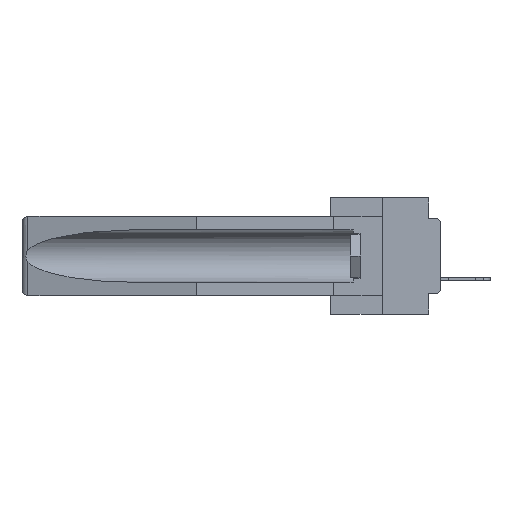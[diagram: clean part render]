
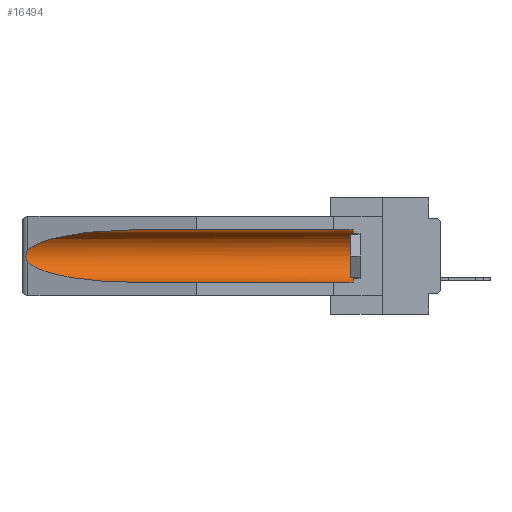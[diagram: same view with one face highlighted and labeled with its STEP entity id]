
A CAD part, left-side view. The second image highlights one B-rep face of the part: STEP entity #16494.
In plain terms, the highlighted cylindrical face has radius 2.857 mm (diameter 5.715 mm), a partial arc.
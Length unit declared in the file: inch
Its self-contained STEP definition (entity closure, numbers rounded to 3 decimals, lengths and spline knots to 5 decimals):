
#127 = CARTESIAN_POINT ( 'NONE',  ( 0.155, 1.07973, -0.284 ) ) ;
#225 = CARTESIAN_POINT ( 'NONE',  ( 0.2673, 1.53269, -0.17917 ) ) ;
#530 = CARTESIAN_POINT ( 'NONE',  ( 0.155, -0.30754, -0.284 ) ) ;
#1042 = ORIENTED_EDGE ( 'NONE', *, *, #26221, .T. ) ;
#1314 = CARTESIAN_POINT ( 'NONE',  ( 0.155, 1.07973, -0.059 ) ) ;
#2080 = ORIENTED_EDGE ( 'NONE', *, *, #26240, .T. ) ;
#2607 = DIRECTION ( 'NONE',  ( 0., 1., 0. ) ) ;
#2804 = CARTESIAN_POINT ( 'NONE',  ( 0.26655, 1.53094, -0.18657 ) ) ;
#3484 = AXIS2_PLACEMENT_3D ( 'NONE', #12619, #2607, #5133 ) ;
#3727 = LINE ( 'NONE', #530, #7672 ) ;
#3952 = ORIENTED_EDGE ( 'NONE', *, *, #25213, .T. ) ;
#4207 = CARTESIAN_POINT ( 'NONE',  ( 0.155, 1.07973, -0.284 ) ) ;
#4616 = VERTEX_POINT ( 'NONE', #1314 ) ;
#5133 = DIRECTION ( 'NONE',  ( 0., 0., 1. ) ) ;
#5212 = CARTESIAN_POINT ( 'NONE',  ( 0.26537, 1.52718, -0.19328 ) ) ;
#5871 = VERTEX_POINT ( 'NONE', #17698 ) ;
#6593 = CYLINDRICAL_SURFACE ( 'NONE', #3484, 0.1125 ) ;
#7661 = LINE ( 'NONE', #12620, #10044 ) ;
#7672 = VECTOR ( 'NONE', #8139, 39.37008 ) ;
#7753 = CARTESIAN_POINT ( 'NONE',  ( 0.26537, 1.52718, -0.14972 ) ) ;
#8139 = DIRECTION ( 'NONE',  ( 0., 1., 0. ) ) ;
#8793 = EDGE_CURVE ( 'NONE', #29252, #5871, #8916, .T. ) ;
#8916 = CIRCLE ( 'NONE', #28473, 0.1125 ) ;
#9761 = CARTESIAN_POINT ( 'NONE',  ( 0.26537, 1.52718, -0.14972 ) ) ;
#9970 = CARTESIAN_POINT ( 'NONE',  ( 0.2673, 1.5327, -0.16383 ) ) ;
#9971 = CARTESIAN_POINT ( 'NONE',  ( 0.25451, 1.48313, -0.24835 ) ) ;
#9983 = CARTESIAN_POINT ( 'NONE',  ( 0.155, 1.07973, -0.059 ) ) ;
#10044 = VECTOR ( 'NONE', #17809, 39.37008 ) ;
#10397 = CARTESIAN_POINT ( 'NONE',  ( 0.25451, 1.48313, -0.09465 ) ) ;
#10589 = CARTESIAN_POINT ( 'NONE',  ( 0.2675, 1.53308, -0.17534 ) ) ;
#11456 = VERTEX_POINT ( 'NONE', #11634 ) ;
#11634 = CARTESIAN_POINT ( 'NONE',  ( 0.26537, 1.52718, -0.14972 ) ) ;
#12619 = CARTESIAN_POINT ( 'NONE',  ( 0.155, -0.30754, -0.1715 ) ) ;
#12620 = CARTESIAN_POINT ( 'NONE',  ( 0.155, -0.30754, -0.059 ) ) ;
#12919 = CARTESIAN_POINT ( 'NONE',  ( 0.26537, 1.52718, -0.19328 ) ) ;
#13600 = B_SPLINE_CURVE_WITH_KNOTS ( 'NONE', 3,
 ( #9761, #22513, #29996, #9970, #27573, #10589, #225, #2804, #22930, #12919 ),
 .UNSPECIFIED., .F., .F.,
 ( 4, 2, 2, 2, 4 ),
 ( 0., 0.00029, 0.00058, 0.00087, 0.00117 ),
 .UNSPECIFIED. ) ;
#15367 = CARTESIAN_POINT ( 'NONE',  ( 0.21114, 1.30732, -0.059 ) ) ;
#15533 = CARTESIAN_POINT ( 'NONE',  ( 0.155, 0.126, -0.284 ) ) ;
#16335 = CARTESIAN_POINT ( 'NONE',  ( 0.26537, 1.52718, -0.19328 ) ) ;
#16494 = ADVANCED_FACE ( 'NONE', ( #31794 ), #6593, .F. ) ;
#17324 = CARTESIAN_POINT ( 'NONE',  ( 0.155, 0.126, -0.1715 ) ) ;
#17591 = CARTESIAN_POINT ( 'NONE',  ( 0.21114, 1.30732, -0.284 ) ) ;
#17698 = CARTESIAN_POINT ( 'NONE',  ( 0.155, 0.126, -0.059 ) ) ;
#17809 = DIRECTION ( 'NONE',  ( 0., 1., 0. ) ) ;
#18340 = ORIENTED_EDGE ( 'NONE', *, *, #21944, .F. ) ;
#19452 =( BOUNDED_CURVE ( )  B_SPLINE_CURVE ( 3, ( #9983, #15367, #10397, #7753 ),
 .UNSPECIFIED., .F., .F. ) 
 B_SPLINE_CURVE_WITH_KNOTS ( ( 4, 4 ),
 ( 4.71239, 6.08839 ),
 .UNSPECIFIED. ) 
 CURVE ( )  GEOMETRIC_REPRESENTATION_ITEM ( )  RATIONAL_B_SPLINE_CURVE ( ( 1., 0.848, 0.848, 1. ) ) 
 REPRESENTATION_ITEM ( '' )  );
#19838 = DIRECTION ( 'NONE',  ( 0., 0., 1. ) ) ;
#20239 = ORIENTED_EDGE ( 'NONE', *, *, #8793, .T. ) ;
#21239 = EDGE_LOOP ( 'NONE', ( #1042, #31362, #3952, #18340, #20239, #2080 ) ) ;
#21944 = EDGE_CURVE ( 'NONE', #29252, #22148, #3727, .T. ) ;
#22148 = VERTEX_POINT ( 'NONE', #4207 ) ;
#22479 = DIRECTION ( 'NONE',  ( 0., -1., 0. ) ) ;
#22513 = CARTESIAN_POINT ( 'NONE',  ( 0.26597, 1.52961, -0.15275 ) ) ;
#22930 = CARTESIAN_POINT ( 'NONE',  ( 0.26597, 1.5296, -0.19026 ) ) ;
#25213 = EDGE_CURVE ( 'NONE', #28925, #22148, #27729, .T. ) ;
#26221 = EDGE_CURVE ( 'NONE', #4616, #11456, #19452, .T. ) ;
#26240 = EDGE_CURVE ( 'NONE', #5871, #4616, #7661, .T. ) ;
#27573 = CARTESIAN_POINT ( 'NONE',  ( 0.2675, 1.53308, -0.16763 ) ) ;
#27729 =( BOUNDED_CURVE ( )  B_SPLINE_CURVE ( 3, ( #5212, #9971, #17591, #127 ),
 .UNSPECIFIED., .F., .F. ) 
 B_SPLINE_CURVE_WITH_KNOTS ( ( 4, 4 ),
 ( 0.1948, 1.5708 ),
 .UNSPECIFIED. ) 
 CURVE ( )  GEOMETRIC_REPRESENTATION_ITEM ( )  RATIONAL_B_SPLINE_CURVE ( ( 1., 0.848, 0.848, 1. ) ) 
 REPRESENTATION_ITEM ( '' )  );
#28473 = AXIS2_PLACEMENT_3D ( 'NONE', #17324, #22479, #19838 ) ;
#28596 = EDGE_CURVE ( 'NONE', #11456, #28925, #13600, .T. ) ;
#28925 = VERTEX_POINT ( 'NONE', #16335 ) ;
#29252 = VERTEX_POINT ( 'NONE', #15533 ) ;
#29996 = CARTESIAN_POINT ( 'NONE',  ( 0.26654, 1.53092, -0.15636 ) ) ;
#31362 = ORIENTED_EDGE ( 'NONE', *, *, #28596, .T. ) ;
#31794 = FACE_OUTER_BOUND ( 'NONE', #21239, .T. ) ;
